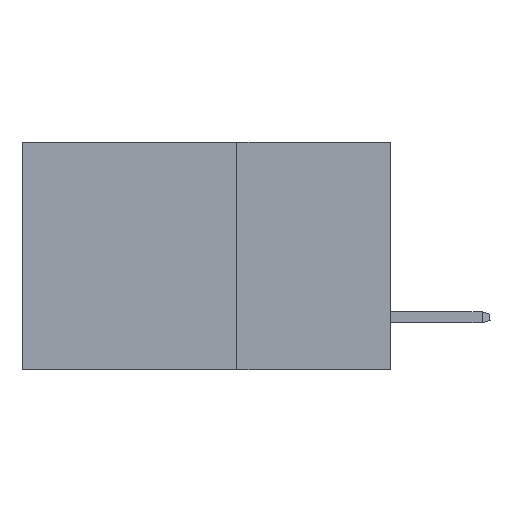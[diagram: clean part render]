
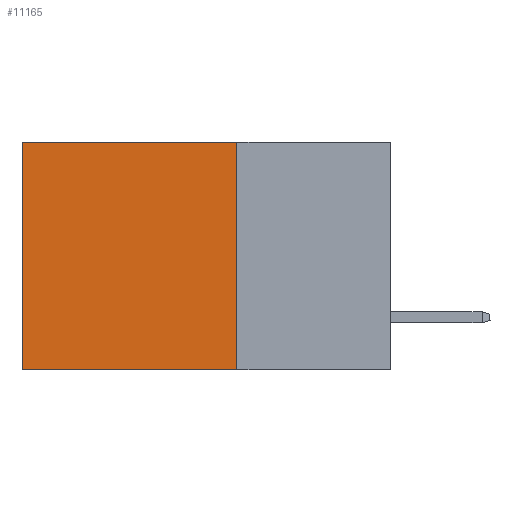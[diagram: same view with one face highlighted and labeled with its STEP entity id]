
A CAD part, left-side view. The second image highlights one B-rep face of the part: STEP entity #11165.
In plain terms, the highlighted planar face has unit normal (-1, 0, 0).
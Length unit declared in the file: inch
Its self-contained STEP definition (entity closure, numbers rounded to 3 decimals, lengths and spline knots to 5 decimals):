
#277 = CARTESIAN_POINT ( 'NONE',  ( 0.2875, 0.25, 0. ) ) ;
#716 = VECTOR ( 'NONE', #8963, 39.37008 ) ;
#1825 = LINE ( 'NONE', #277, #22690 ) ;
#2261 = VERTEX_POINT ( 'NONE', #10677 ) ;
#2679 = EDGE_CURVE ( 'NONE', #15201, #47123, #10872, .T. ) ;
#4412 = PLANE ( 'NONE',  #46588 ) ;
#5333 = CARTESIAN_POINT ( 'NONE',  ( 0.2875, 0.6, -0.37 ) ) ;
#8963 = DIRECTION ( 'NONE',  ( 0., 1., 0. ) ) ;
#10677 = CARTESIAN_POINT ( 'NONE',  ( 0.2875, 0.25, 0. ) ) ;
#10872 = LINE ( 'NONE', #21107, #716 ) ;
#11165 = ADVANCED_FACE ( 'NONE', ( #44162 ), #4412, .F. ) ;
#11302 = DIRECTION ( 'NONE',  ( 0., 0., -1. ) ) ;
#11626 = CARTESIAN_POINT ( 'NONE',  ( 0.2875, 0.6, 0. ) ) ;
#11949 = ORIENTED_EDGE ( 'NONE', *, *, #28157, .F. ) ;
#12707 = EDGE_LOOP ( 'NONE', ( #16002, #37743, #11949, #21228 ) ) ;
#15201 = VERTEX_POINT ( 'NONE', #30397 ) ;
#15930 = DIRECTION ( 'NONE',  ( 0., 0., -1. ) ) ;
#15945 = VECTOR ( 'NONE', #15930, 39.37008 ) ;
#16002 = ORIENTED_EDGE ( 'NONE', *, *, #23215, .T. ) ;
#16364 = CARTESIAN_POINT ( 'NONE',  ( 0.2875, 0.6, 0. ) ) ;
#19234 = DIRECTION ( 'NONE',  ( 0., 0., -1. ) ) ;
#21107 = CARTESIAN_POINT ( 'NONE',  ( 0.2875, 0.25, -0.37 ) ) ;
#21228 = ORIENTED_EDGE ( 'NONE', *, *, #45347, .T. ) ;
#22013 = VERTEX_POINT ( 'NONE', #16364 ) ;
#22690 = VECTOR ( 'NONE', #38717, 39.37008 ) ;
#22867 = CARTESIAN_POINT ( 'NONE',  ( 0.2875, 0.25, 0. ) ) ;
#23215 = EDGE_CURVE ( 'NONE', #22013, #47123, #42092, .T. ) ;
#28157 = EDGE_CURVE ( 'NONE', #2261, #15201, #46100, .T. ) ;
#30397 = CARTESIAN_POINT ( 'NONE',  ( 0.2875, 0.25, -0.37 ) ) ;
#37743 = ORIENTED_EDGE ( 'NONE', *, *, #2679, .F. ) ;
#38544 = CARTESIAN_POINT ( 'NONE',  ( 0.2875, 0.25, 0. ) ) ;
#38717 = DIRECTION ( 'NONE',  ( 0., 1., 0. ) ) ;
#41803 = DIRECTION ( 'NONE',  ( 1., 0., 0. ) ) ;
#42092 = LINE ( 'NONE', #11626, #47444 ) ;
#44162 = FACE_OUTER_BOUND ( 'NONE', #12707, .T. ) ;
#45347 = EDGE_CURVE ( 'NONE', #2261, #22013, #1825, .T. ) ;
#46100 = LINE ( 'NONE', #38544, #15945 ) ;
#46588 = AXIS2_PLACEMENT_3D ( 'NONE', #22867, #41803, #19234 ) ;
#47123 = VERTEX_POINT ( 'NONE', #5333 ) ;
#47444 = VECTOR ( 'NONE', #11302, 39.37008 ) ;
